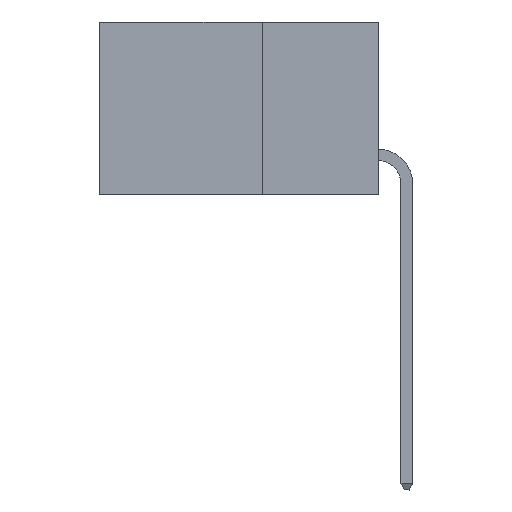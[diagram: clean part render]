
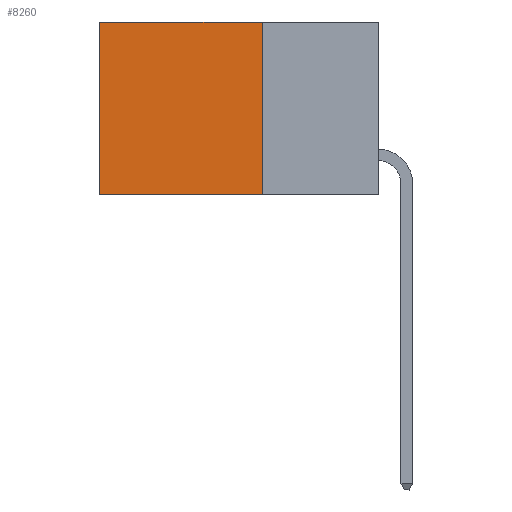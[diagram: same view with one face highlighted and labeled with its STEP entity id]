
A CAD part, left-side view. The second image highlights one B-rep face of the part: STEP entity #8260.
In plain terms, the highlighted planar face has unit normal (-1, 0, 0).
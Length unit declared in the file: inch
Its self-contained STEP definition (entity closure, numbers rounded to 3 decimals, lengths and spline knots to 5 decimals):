
#7 = CARTESIAN_POINT ( 'NONE',  ( 0.298, 0.25, 0. ) ) ;
#590 = EDGE_CURVE ( 'NONE', #12646, #4352, #12802, .T. ) ;
#731 = VECTOR ( 'NONE', #7701, 39.37008 ) ;
#1089 = DIRECTION ( 'NONE',  ( 0., 0., -1. ) ) ;
#1109 = CARTESIAN_POINT ( 'NONE',  ( 0.298, 0.25, -0.37 ) ) ;
#1207 = CARTESIAN_POINT ( 'NONE',  ( 0.298, 0.6, 0. ) ) ;
#1618 = VECTOR ( 'NONE', #10202, 39.37008 ) ;
#2070 = CARTESIAN_POINT ( 'NONE',  ( 0.298, 0.25, -0.37 ) ) ;
#3294 = CARTESIAN_POINT ( 'NONE',  ( 0.298, 0.6, -0.37 ) ) ;
#3316 = PLANE ( 'NONE',  #7973 ) ;
#3353 = VERTEX_POINT ( 'NONE', #1207 ) ;
#3582 = CARTESIAN_POINT ( 'NONE',  ( 0.298, 0.6, 0. ) ) ;
#4234 = CARTESIAN_POINT ( 'NONE',  ( 0.298, 0.25, 0. ) ) ;
#4352 = VERTEX_POINT ( 'NONE', #1109 ) ;
#4839 = EDGE_LOOP ( 'NONE', ( #8368, #5123, #11277, #10902 ) ) ;
#5123 = ORIENTED_EDGE ( 'NONE', *, *, #5470, .F. ) ;
#5162 = VECTOR ( 'NONE', #6989, 39.37008 ) ;
#5470 = EDGE_CURVE ( 'NONE', #4352, #6000, #11043, .T. ) ;
#6000 = VERTEX_POINT ( 'NONE', #3294 ) ;
#6068 = EDGE_CURVE ( 'NONE', #3353, #6000, #7828, .T. ) ;
#6989 = DIRECTION ( 'NONE',  ( 0., 0., -1. ) ) ;
#7575 = EDGE_CURVE ( 'NONE', #12646, #3353, #10823, .T. ) ;
#7701 = DIRECTION ( 'NONE',  ( 0., 1., 0. ) ) ;
#7828 = LINE ( 'NONE', #3582, #5162 ) ;
#7973 = AXIS2_PLACEMENT_3D ( 'NONE', #7, #14733, #1089 ) ;
#8260 = ADVANCED_FACE ( 'NONE', ( #11532 ), #3316, .F. ) ;
#8368 = ORIENTED_EDGE ( 'NONE', *, *, #6068, .T. ) ;
#9804 = VECTOR ( 'NONE', #9879, 39.37008 ) ;
#9879 = DIRECTION ( 'NONE',  ( 0., 1., 0. ) ) ;
#10202 = DIRECTION ( 'NONE',  ( 0., 0., -1. ) ) ;
#10823 = LINE ( 'NONE', #4234, #731 ) ;
#10902 = ORIENTED_EDGE ( 'NONE', *, *, #7575, .T. ) ;
#11043 = LINE ( 'NONE', #2070, #9804 ) ;
#11277 = ORIENTED_EDGE ( 'NONE', *, *, #590, .F. ) ;
#11532 = FACE_OUTER_BOUND ( 'NONE', #4839, .T. ) ;
#12601 = CARTESIAN_POINT ( 'NONE',  ( 0.298, 0.25, 0. ) ) ;
#12646 = VERTEX_POINT ( 'NONE', #12601 ) ;
#12802 = LINE ( 'NONE', #13610, #1618 ) ;
#13610 = CARTESIAN_POINT ( 'NONE',  ( 0.298, 0.25, 0. ) ) ;
#14733 = DIRECTION ( 'NONE',  ( 1., 0., 0. ) ) ;
